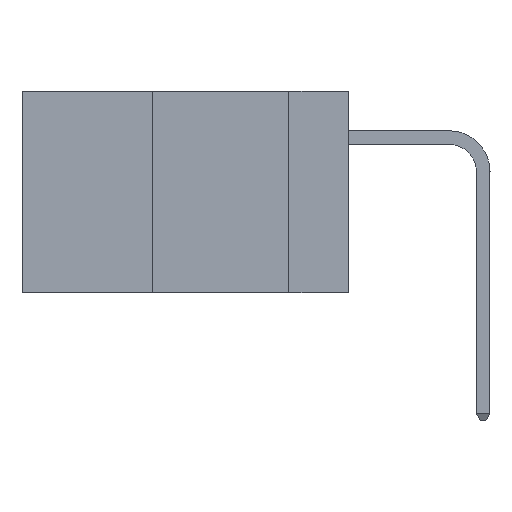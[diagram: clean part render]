
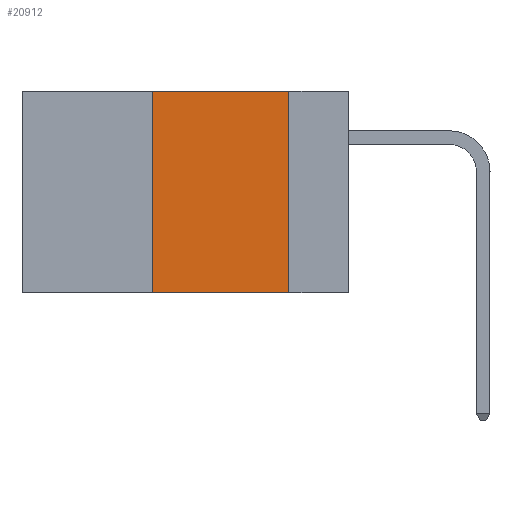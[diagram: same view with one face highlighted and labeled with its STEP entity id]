
A CAD part, left-side view. The second image highlights one B-rep face of the part: STEP entity #20912.
In plain terms, the highlighted planar face has unit normal (-1, 0, 0).
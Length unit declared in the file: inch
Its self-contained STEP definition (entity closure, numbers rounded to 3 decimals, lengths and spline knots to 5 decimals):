
#1334 = FACE_OUTER_BOUND ( 'NONE', #11348, .T. ) ;
#1718 = VERTEX_POINT ( 'NONE', #14331 ) ;
#3155 = LINE ( 'NONE', #21324, #17452 ) ;
#3228 = DIRECTION ( 'NONE',  ( 1., 0., 0. ) ) ;
#3967 = EDGE_CURVE ( 'NONE', #1718, #6052, #7584, .T. ) ;
#4053 = VERTEX_POINT ( 'NONE', #20302 ) ;
#4958 = ORIENTED_EDGE ( 'NONE', *, *, #3967, .F. ) ;
#5793 = CARTESIAN_POINT ( 'NONE',  ( 0., 0.6, 0. ) ) ;
#6052 = VERTEX_POINT ( 'NONE', #10338 ) ;
#6062 = EDGE_CURVE ( 'NONE', #6052, #6692, #3155, .T. ) ;
#6084 = EDGE_CURVE ( 'NONE', #4053, #1718, #8760, .T. ) ;
#6692 = VERTEX_POINT ( 'NONE', #12888 ) ;
#7584 = LINE ( 'NONE', #5793, #13180 ) ;
#8304 = AXIS2_PLACEMENT_3D ( 'NONE', #19262, #3228, #14229 ) ;
#8412 = EDGE_CURVE ( 'NONE', #4053, #6692, #21998, .T. ) ;
#8478 = VECTOR ( 'NONE', #11250, 39.37008 ) ;
#8760 = LINE ( 'NONE', #23119, #12860 ) ;
#9023 = ORIENTED_EDGE ( 'NONE', *, *, #6084, .F. ) ;
#9092 = CARTESIAN_POINT ( 'NONE',  ( 0., 0.6, -0.37 ) ) ;
#10212 = DIRECTION ( 'NONE',  ( 0., 0., 1. ) ) ;
#10338 = CARTESIAN_POINT ( 'NONE',  ( 0., 0.11, 0. ) ) ;
#10706 = ORIENTED_EDGE ( 'NONE', *, *, #6062, .F. ) ;
#11250 = DIRECTION ( 'NONE',  ( 0., -1., 0. ) ) ;
#11348 = EDGE_LOOP ( 'NONE', ( #10706, #4958, #9023, #22954 ) ) ;
#12860 = VECTOR ( 'NONE', #10212, 39.37008 ) ;
#12888 = CARTESIAN_POINT ( 'NONE',  ( 0., 0.11, -0.37 ) ) ;
#13088 = DIRECTION ( 'NONE',  ( 0., -1., 0. ) ) ;
#13180 = VECTOR ( 'NONE', #13088, 39.37008 ) ;
#14229 = DIRECTION ( 'NONE',  ( 0., 0., -1. ) ) ;
#14331 = CARTESIAN_POINT ( 'NONE',  ( 0., 0.36, 0. ) ) ;
#15946 = DIRECTION ( 'NONE',  ( 0., 0., -1. ) ) ;
#17452 = VECTOR ( 'NONE', #15946, 39.37008 ) ;
#19262 = CARTESIAN_POINT ( 'NONE',  ( 0., 0.6, 0. ) ) ;
#20302 = CARTESIAN_POINT ( 'NONE',  ( 0., 0.36, -0.37 ) ) ;
#20912 = ADVANCED_FACE ( 'NONE', ( #1334 ), #22855, .F. ) ;
#21324 = CARTESIAN_POINT ( 'NONE',  ( 0., 0.11, 0. ) ) ;
#21998 = LINE ( 'NONE', #9092, #8478 ) ;
#22855 = PLANE ( 'NONE',  #8304 ) ;
#22954 = ORIENTED_EDGE ( 'NONE', *, *, #8412, .T. ) ;
#23119 = CARTESIAN_POINT ( 'NONE',  ( 0., 0.36, 0. ) ) ;
